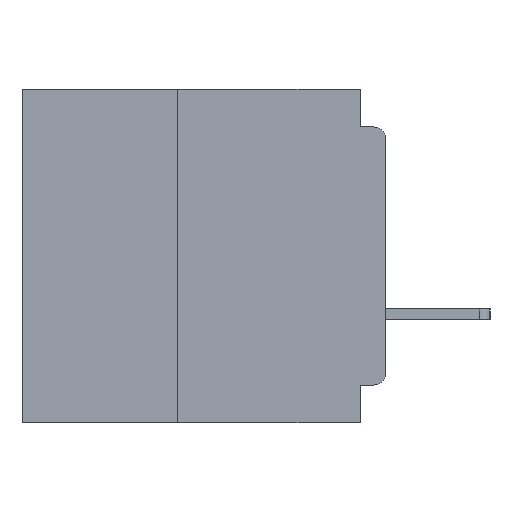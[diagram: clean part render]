
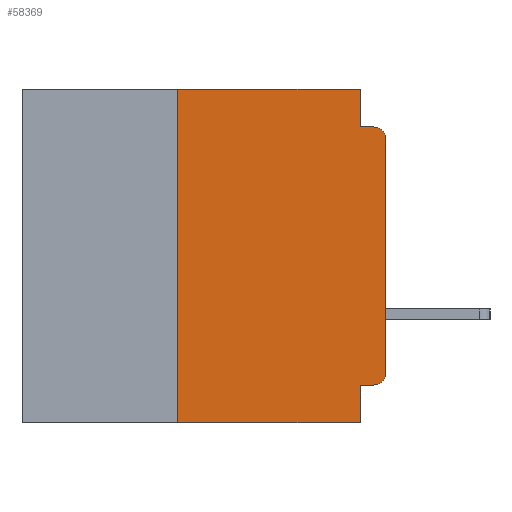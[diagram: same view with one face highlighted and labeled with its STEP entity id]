
A CAD part, left-side view. The second image highlights one B-rep face of the part: STEP entity #58369.
In plain terms, the highlighted planar face has unit normal (-1, 0, 0).
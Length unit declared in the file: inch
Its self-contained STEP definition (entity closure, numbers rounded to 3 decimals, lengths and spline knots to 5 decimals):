
#155 = CARTESIAN_POINT ( 'NONE',  ( 0., 0., -0.34 ) ) ;
#2820 = CARTESIAN_POINT ( 'NONE',  ( 0., 0.031, -0.045 ) ) ;
#3691 = ORIENTED_EDGE ( 'NONE', *, *, #52872, .F. ) ;
#5399 = VERTEX_POINT ( 'NONE', #13316 ) ;
#5543 = EDGE_CURVE ( 'NONE', #9908, #63311, #40253, .T. ) ;
#5695 = ORIENTED_EDGE ( 'NONE', *, *, #5543, .F. ) ;
#6599 = EDGE_CURVE ( 'NONE', #25828, #49466, #37673, .T. ) ;
#7392 = VECTOR ( 'NONE', #21959, 39.37008 ) ;
#9908 = VERTEX_POINT ( 'NONE', #52596 ) ;
#10156 = LINE ( 'NONE', #46235, #63289 ) ;
#10374 = VECTOR ( 'NONE', #38372, 39.37008 ) ;
#10925 = ORIENTED_EDGE ( 'NONE', *, *, #13408, .F. ) ;
#11691 = DIRECTION ( 'NONE',  ( 1., 0., 0. ) ) ;
#12538 = CARTESIAN_POINT ( 'NONE',  ( 0., 0.031, -0.355 ) ) ;
#12677 = CARTESIAN_POINT ( 'NONE',  ( 0., 0.25, 0. ) ) ;
#12785 = CARTESIAN_POINT ( 'NONE',  ( 0., 0., 0. ) ) ;
#13101 = VERTEX_POINT ( 'NONE', #12677 ) ;
#13316 = CARTESIAN_POINT ( 'NONE',  ( 0., 0.25, -0.4 ) ) ;
#13408 = EDGE_CURVE ( 'NONE', #5399, #13101, #24641, .T. ) ;
#13509 = VECTOR ( 'NONE', #16484, 39.37008 ) ;
#15132 = LINE ( 'NONE', #57700, #13509 ) ;
#15465 = DIRECTION ( 'NONE',  ( 0., -1., 0. ) ) ;
#15808 = ORIENTED_EDGE ( 'NONE', *, *, #49195, .F. ) ;
#16484 = DIRECTION ( 'NONE',  ( 0., 0., -1. ) ) ;
#19854 = AXIS2_PLACEMENT_3D ( 'NONE', #60073, #29101, #65152 ) ;
#20154 = ORIENTED_EDGE ( 'NONE', *, *, #21077, .T. ) ;
#21077 = EDGE_CURVE ( 'NONE', #49466, #65165, #38035, .T. ) ;
#21778 = CARTESIAN_POINT ( 'NONE',  ( 0., 0.437, 0. ) ) ;
#21959 = DIRECTION ( 'NONE',  ( 0., -1., 0. ) ) ;
#23703 = CARTESIAN_POINT ( 'NONE',  ( 0., 0.015, -0.045 ) ) ;
#24641 = LINE ( 'NONE', #61468, #55357 ) ;
#24972 = CARTESIAN_POINT ( 'NONE',  ( 0., 0.015, -0.06 ) ) ;
#25472 = CARTESIAN_POINT ( 'NONE',  ( 0., 0.437, 0. ) ) ;
#25828 = VERTEX_POINT ( 'NONE', #155 ) ;
#27361 = LINE ( 'NONE', #30232, #54887 ) ;
#28373 = AXIS2_PLACEMENT_3D ( 'NONE', #21778, #11691, #47657 ) ;
#28656 = EDGE_CURVE ( 'NONE', #13101, #38282, #48825, .T. ) ;
#28722 = ORIENTED_EDGE ( 'NONE', *, *, #28656, .F. ) ;
#29101 = DIRECTION ( 'NONE',  ( -1., 0., 0. ) ) ;
#30120 = DIRECTION ( 'NONE',  ( 0., 0., -1. ) ) ;
#30232 = CARTESIAN_POINT ( 'NONE',  ( 0., 0.031, 0. ) ) ;
#32677 = ORIENTED_EDGE ( 'NONE', *, *, #6599, .T. ) ;
#34136 = CARTESIAN_POINT ( 'NONE',  ( 0., 0., -0.06 ) ) ;
#34666 = LINE ( 'NONE', #37231, #7392 ) ;
#35040 = VECTOR ( 'NONE', #46211, 39.37008 ) ;
#35378 = VERTEX_POINT ( 'NONE', #2820 ) ;
#35431 = DIRECTION ( 'NONE',  ( 0., 0., -1. ) ) ;
#37231 = CARTESIAN_POINT ( 'NONE',  ( 0., 0.437, -0.4 ) ) ;
#37673 = LINE ( 'NONE', #12785, #10374 ) ;
#38035 = CIRCLE ( 'NONE', #57663, 0.015 ) ;
#38282 = VERTEX_POINT ( 'NONE', #56868 ) ;
#38372 = DIRECTION ( 'NONE',  ( 0., 0., 1. ) ) ;
#40253 = LINE ( 'NONE', #50454, #52440 ) ;
#40516 = EDGE_CURVE ( 'NONE', #35378, #65165, #10156, .T. ) ;
#40931 = VERTEX_POINT ( 'NONE', #44374 ) ;
#41091 = FACE_OUTER_BOUND ( 'NONE', #46207, .T. ) ;
#42316 = CIRCLE ( 'NONE', #19854, 0.015 ) ;
#42431 = PLANE ( 'NONE',  #28373 ) ;
#42605 = ORIENTED_EDGE ( 'NONE', *, *, #40516, .F. ) ;
#44374 = CARTESIAN_POINT ( 'NONE',  ( 0., 0.031, -0.4 ) ) ;
#45889 = DIRECTION ( 'NONE',  ( 0., 0., 1. ) ) ;
#46207 = EDGE_LOOP ( 'NONE', ( #32677, #20154, #42605, #3691, #28722, #10925, #50144, #15808, #5695, #65574 ) ) ;
#46211 = DIRECTION ( 'NONE',  ( 0., -1., 0. ) ) ;
#46235 = CARTESIAN_POINT ( 'NONE',  ( 0., 0., -0.045 ) ) ;
#47657 = DIRECTION ( 'NONE',  ( 0., 0., -1. ) ) ;
#48825 = LINE ( 'NONE', #25472, #35040 ) ;
#49195 = EDGE_CURVE ( 'NONE', #63311, #40931, #15132, .T. ) ;
#49466 = VERTEX_POINT ( 'NONE', #34136 ) ;
#49991 = EDGE_CURVE ( 'NONE', #9908, #25828, #42316, .T. ) ;
#50144 = ORIENTED_EDGE ( 'NONE', *, *, #63193, .T. ) ;
#50454 = CARTESIAN_POINT ( 'NONE',  ( 0., 0., -0.355 ) ) ;
#52440 = VECTOR ( 'NONE', #55655, 39.37008 ) ;
#52596 = CARTESIAN_POINT ( 'NONE',  ( 0., 0.015, -0.355 ) ) ;
#52872 = EDGE_CURVE ( 'NONE', #38282, #35378, #27361, .T. ) ;
#54887 = VECTOR ( 'NONE', #35431, 39.37008 ) ;
#55357 = VECTOR ( 'NONE', #45889, 39.37008 ) ;
#55655 = DIRECTION ( 'NONE',  ( 0., 1., 0. ) ) ;
#56868 = CARTESIAN_POINT ( 'NONE',  ( 0., 0.031, 0. ) ) ;
#57663 = AXIS2_PLACEMENT_3D ( 'NONE', #24972, #61057, #30120 ) ;
#57700 = CARTESIAN_POINT ( 'NONE',  ( 0., 0.031, -0.4 ) ) ;
#58369 = ADVANCED_FACE ( 'NONE', ( #41091 ), #42431, .F. ) ;
#60073 = CARTESIAN_POINT ( 'NONE',  ( 0., 0.015, -0.34 ) ) ;
#61057 = DIRECTION ( 'NONE',  ( -1., 0., 0. ) ) ;
#61468 = CARTESIAN_POINT ( 'NONE',  ( 0., 0.25, -0.4 ) ) ;
#63193 = EDGE_CURVE ( 'NONE', #5399, #40931, #34666, .T. ) ;
#63289 = VECTOR ( 'NONE', #15465, 39.37008 ) ;
#63311 = VERTEX_POINT ( 'NONE', #12538 ) ;
#65152 = DIRECTION ( 'NONE',  ( 0., 0., -1. ) ) ;
#65165 = VERTEX_POINT ( 'NONE', #23703 ) ;
#65574 = ORIENTED_EDGE ( 'NONE', *, *, #49991, .T. ) ;
